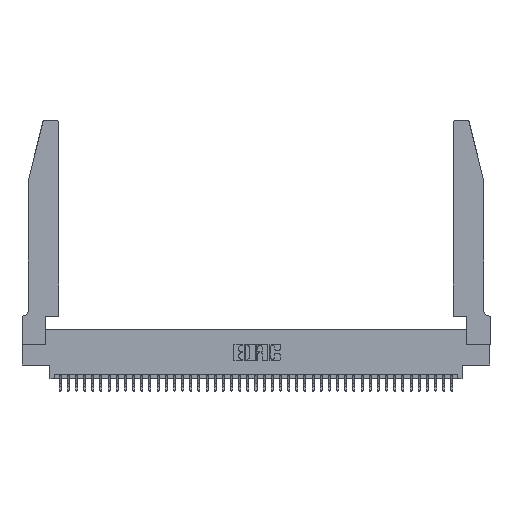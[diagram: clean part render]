
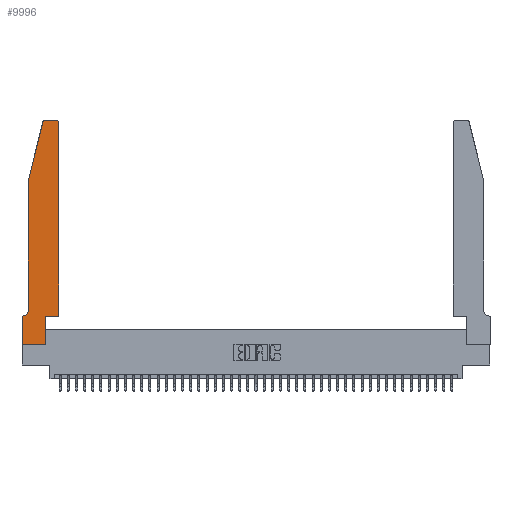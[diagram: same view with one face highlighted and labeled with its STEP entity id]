
A CAD part, top view. The second image highlights one B-rep face of the part: STEP entity #9996.
In plain terms, the highlighted planar face has unit normal (0, 0, 1).
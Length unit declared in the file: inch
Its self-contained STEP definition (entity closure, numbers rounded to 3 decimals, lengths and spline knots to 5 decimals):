
#311 = VECTOR ( 'NONE', #31275, 39.37008 ) ;
#381 = ORIENTED_EDGE ( 'NONE', *, *, #32415, .T. ) ;
#836 = CARTESIAN_POINT ( 'NONE',  ( 0., 0., 0.37 ) ) ;
#1332 = EDGE_CURVE ( 'NONE', #29532, #26407, #16306, .T. ) ;
#1357 = CIRCLE ( 'NONE', #24953, 0.07 ) ;
#1450 = EDGE_CURVE ( 'NONE', #19520, #20746, #26120, .T. ) ;
#1609 = VECTOR ( 'NONE', #28983, 39.37008 ) ;
#2316 = VERTEX_POINT ( 'NONE', #18710 ) ;
#2699 = EDGE_CURVE ( 'NONE', #36529, #29532, #32673, .T. ) ;
#2815 = ORIENTED_EDGE ( 'NONE', *, *, #15381, .T. ) ;
#3594 = CARTESIAN_POINT ( 'NONE',  ( 0.0055, 0.42, 0.37 ) ) ;
#3597 = ORIENTED_EDGE ( 'NONE', *, *, #1450, .T. ) ;
#3863 = DIRECTION ( 'NONE',  ( 0., -1., 0. ) ) ;
#6731 = DIRECTION ( 'NONE',  ( -0.239, -0.971, 0. ) ) ;
#7318 = ORIENTED_EDGE ( 'NONE', *, *, #35775, .T. ) ;
#7487 = DIRECTION ( 'NONE',  ( 0., 0., 1. ) ) ;
#8792 = AXIS2_PLACEMENT_3D ( 'NONE', #13736, #36736, #17039 ) ;
#8974 = CARTESIAN_POINT ( 'NONE',  ( 0., 0., 0.37 ) ) ;
#9050 = EDGE_CURVE ( 'NONE', #33375, #19520, #36975, .T. ) ;
#9105 = LINE ( 'NONE', #836, #22306 ) ;
#9435 = PLANE ( 'NONE',  #30713 ) ;
#9536 = CARTESIAN_POINT ( 'NONE',  ( 0.4505, 0.35, 0.37 ) ) ;
#9685 = VERTEX_POINT ( 'NONE', #32677 ) ;
#9925 = EDGE_CURVE ( 'NONE', #30229, #2316, #21518, .T. ) ;
#9996 = ADVANCED_FACE ( 'NONE', ( #36376 ), #9435, .T. ) ;
#10179 = DIRECTION ( 'NONE',  ( 0., 1., 0. ) ) ;
#11566 = VECTOR ( 'NONE', #10179, 39.37008 ) ;
#13152 = DIRECTION ( 'NONE',  ( -1., 0., 0. ) ) ;
#13321 = LINE ( 'NONE', #17500, #31326 ) ;
#13736 = CARTESIAN_POINT ( 'NONE',  ( 0.284, 2.72, 0.37 ) ) ;
#13779 = ORIENTED_EDGE ( 'NONE', *, *, #9050, .T. ) ;
#13838 = LINE ( 'NONE', #34388, #21601 ) ;
#14143 = CARTESIAN_POINT ( 'NONE',  ( 0.2865, 0.35, 0.37 ) ) ;
#14577 = EDGE_LOOP ( 'NONE', ( #3597, #17843, #33404, #30237, #29960, #381, #33263, #28778, #2815, #17758, #7318, #13779 ) ) ;
#14965 = CARTESIAN_POINT ( 'NONE',  ( 0.4205, 2.75, 0.37 ) ) ;
#15381 = EDGE_CURVE ( 'NONE', #2316, #24945, #13321, .T. ) ;
#15451 = DIRECTION ( 'NONE',  ( 1., 0., 0. ) ) ;
#16306 = LINE ( 'NONE', #24829, #311 ) ;
#17039 = DIRECTION ( 'NONE',  ( 1., 0., 0. ) ) ;
#17139 = AXIS2_PLACEMENT_3D ( 'NONE', #27224, #7487, #37093 ) ;
#17500 = CARTESIAN_POINT ( 'NONE',  ( 0.2865, 0.35, 0.37 ) ) ;
#17758 = ORIENTED_EDGE ( 'NONE', *, *, #39271, .T. ) ;
#17843 = ORIENTED_EDGE ( 'NONE', *, *, #38266, .T. ) ;
#18017 = CARTESIAN_POINT ( 'NONE',  ( 0.25487, 2.72718, 0.37 ) ) ;
#18710 = CARTESIAN_POINT ( 'NONE',  ( 0.2865, 0., 0.37 ) ) ;
#19520 = VERTEX_POINT ( 'NONE', #14965 ) ;
#19800 = VERTEX_POINT ( 'NONE', #21440 ) ;
#20437 = VECTOR ( 'NONE', #13152, 39.37008 ) ;
#20746 = VERTEX_POINT ( 'NONE', #38436 ) ;
#20963 = VECTOR ( 'NONE', #20987, 39.37008 ) ;
#20987 = DIRECTION ( 'NONE',  ( 1., 0., 0. ) ) ;
#21031 = DIRECTION ( 'NONE',  ( -1., 0., 0. ) ) ;
#21207 = LINE ( 'NONE', #9536, #1609 ) ;
#21379 = VECTOR ( 'NONE', #6731, 39.37008 ) ;
#21440 = CARTESIAN_POINT ( 'NONE',  ( 0.4505, 0.35, 0.37 ) ) ;
#21518 = LINE ( 'NONE', #22285, #20963 ) ;
#21601 = VECTOR ( 'NONE', #31235, 39.37008 ) ;
#21859 = DIRECTION ( 'NONE',  ( 0., 1., 0. ) ) ;
#22285 = CARTESIAN_POINT ( 'NONE',  ( 0., 0., 0.37 ) ) ;
#22306 = VECTOR ( 'NONE', #3863, 39.37008 ) ;
#22532 = CARTESIAN_POINT ( 'NONE',  ( 0., 0.35, 0.37 ) ) ;
#23285 = CARTESIAN_POINT ( 'NONE',  ( 0.4505, 0.35, 0.37 ) ) ;
#24603 = EDGE_CURVE ( 'NONE', #37028, #30229, #9105, .T. ) ;
#24829 = CARTESIAN_POINT ( 'NONE',  ( 0.0755, 2., 0.37 ) ) ;
#24945 = VERTEX_POINT ( 'NONE', #14143 ) ;
#24953 = AXIS2_PLACEMENT_3D ( 'NONE', #3594, #39982, #21031 ) ;
#25118 = EDGE_CURVE ( 'NONE', #26407, #9685, #1357, .T. ) ;
#26120 = LINE ( 'NONE', #29843, #20437 ) ;
#26407 = VERTEX_POINT ( 'NONE', #37288 ) ;
#26724 = CARTESIAN_POINT ( 'NONE',  ( 0.0755, 2., 0.37 ) ) ;
#27224 = CARTESIAN_POINT ( 'NONE',  ( 0.4205, 2.72, 0.37 ) ) ;
#27232 = CARTESIAN_POINT ( 'NONE',  ( 0., 0.35, 0.37 ) ) ;
#28778 = ORIENTED_EDGE ( 'NONE', *, *, #9925, .T. ) ;
#28875 = DIRECTION ( 'NONE',  ( 0., 0., 1. ) ) ;
#28983 = DIRECTION ( 'NONE',  ( 1., 0., 0. ) ) ;
#29532 = VERTEX_POINT ( 'NONE', #31596 ) ;
#29843 = CARTESIAN_POINT ( 'NONE',  ( 0.2605, 2.75, 0.37 ) ) ;
#29960 = ORIENTED_EDGE ( 'NONE', *, *, #25118, .T. ) ;
#30229 = VERTEX_POINT ( 'NONE', #8974 ) ;
#30237 = ORIENTED_EDGE ( 'NONE', *, *, #1332, .T. ) ;
#30713 = AXIS2_PLACEMENT_3D ( 'NONE', #22532, #28875, #15451 ) ;
#31235 = DIRECTION ( 'NONE',  ( -1., 0., 0. ) ) ;
#31275 = DIRECTION ( 'NONE',  ( 0., -1., 0. ) ) ;
#31326 = VECTOR ( 'NONE', #21859, 39.37008 ) ;
#31596 = CARTESIAN_POINT ( 'NONE',  ( 0.0755, 2., 0.37 ) ) ;
#31604 = LINE ( 'NONE', #23285, #11566 ) ;
#32415 = EDGE_CURVE ( 'NONE', #9685, #37028, #13838, .T. ) ;
#32673 = LINE ( 'NONE', #26724, #21379 ) ;
#32677 = CARTESIAN_POINT ( 'NONE',  ( 0.0055, 0.35, 0.37 ) ) ;
#33263 = ORIENTED_EDGE ( 'NONE', *, *, #24603, .T. ) ;
#33375 = VERTEX_POINT ( 'NONE', #42537 ) ;
#33404 = ORIENTED_EDGE ( 'NONE', *, *, #2699, .T. ) ;
#34147 = CIRCLE ( 'NONE', #8792, 0.03 ) ;
#34388 = CARTESIAN_POINT ( 'NONE',  ( 0.0755, 0.35, 0.37 ) ) ;
#35775 = EDGE_CURVE ( 'NONE', #19800, #33375, #31604, .T. ) ;
#36376 = FACE_OUTER_BOUND ( 'NONE', #14577, .T. ) ;
#36529 = VERTEX_POINT ( 'NONE', #18017 ) ;
#36736 = DIRECTION ( 'NONE',  ( 0., 0., 1. ) ) ;
#36975 = CIRCLE ( 'NONE', #17139, 0.03 ) ;
#37028 = VERTEX_POINT ( 'NONE', #27232 ) ;
#37093 = DIRECTION ( 'NONE',  ( 1., 0., 0. ) ) ;
#37288 = CARTESIAN_POINT ( 'NONE',  ( 0.0755, 0.42, 0.37 ) ) ;
#38266 = EDGE_CURVE ( 'NONE', #20746, #36529, #34147, .T. ) ;
#38436 = CARTESIAN_POINT ( 'NONE',  ( 0.284, 2.75, 0.37 ) ) ;
#39271 = EDGE_CURVE ( 'NONE', #24945, #19800, #21207, .T. ) ;
#39982 = DIRECTION ( 'NONE',  ( 0., 0., -1. ) ) ;
#42537 = CARTESIAN_POINT ( 'NONE',  ( 0.4505, 2.72, 0.37 ) ) ;
